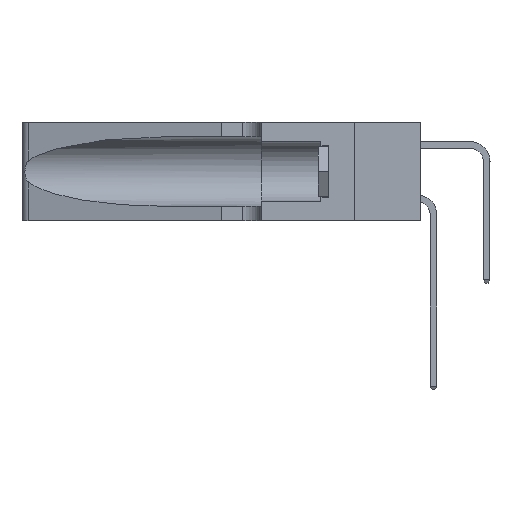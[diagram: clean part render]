
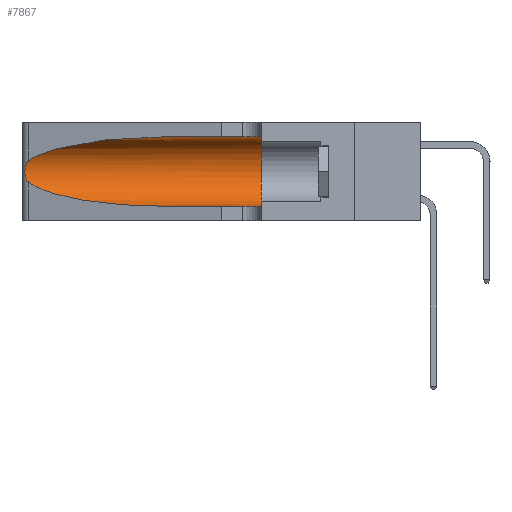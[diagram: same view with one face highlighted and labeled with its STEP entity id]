
A CAD part, left-side view. The second image highlights one B-rep face of the part: STEP entity #7867.
In plain terms, the highlighted cylindrical face has radius 3.308 mm (diameter 6.617 mm), a partial arc.
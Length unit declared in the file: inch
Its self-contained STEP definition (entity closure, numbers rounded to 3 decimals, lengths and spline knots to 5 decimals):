
#115 = CARTESIAN_POINT ( 'NONE',  ( 0.1305, 0.72297, 0.31525 ) ) ;
#390 = B_SPLINE_CURVE_WITH_KNOTS ( 'NONE', 3,
 ( #10693, #12631, #2793, #16438, #4817, #18344, #6835, #20268, #8833, #22129, #10775, #24006, #12704, #839 ),
 .UNSPECIFIED., .F., .F.,
 ( 4, 2, 2, 2, 2, 2, 4 ),
 ( 0., 0.00027, 0.00053, 0.00107, 0.0016, 0.00187, 0.00214 ),
 .UNSPECIFIED. ) ;
#839 = CARTESIAN_POINT ( 'NONE',  ( 0.25487, 1.22718, 0.14631 ) ) ;
#1038 = EDGE_CURVE ( 'NONE', #15591, #4184, #21441, .T. ) ;
#1065 =( BOUNDED_CURVE ( )  B_SPLINE_CURVE ( 3, ( #23646, #10409, #14245, #2492 ),
 .UNSPECIFIED., .F., .T. ) 
 B_SPLINE_CURVE_WITH_KNOTS ( ( 4, 4 ),
 ( 1.5708, 2.84003 ),
 .UNSPECIFIED. ) 
 CURVE ( )  GEOMETRIC_REPRESENTATION_ITEM ( )  RATIONAL_B_SPLINE_CURVE ( ( 1., 0.87, 0.87, 1. ) ) 
 REPRESENTATION_ITEM ( '' )  );
#2492 = CARTESIAN_POINT ( 'NONE',  ( 0.25487, 1.22718, 0.22369 ) ) ;
#2641 = CARTESIAN_POINT ( 'NONE',  ( 0.25487, 1.22718, 0.14631 ) ) ;
#2793 = CARTESIAN_POINT ( 'NONE',  ( 0.25639, 1.23184, 0.21858 ) ) ;
#2945 = DIRECTION ( 'NONE',  ( 0., 0., -1. ) ) ;
#3010 = EDGE_LOOP ( 'NONE', ( #16936, #16941, #18572, #11114, #23501, #21660 ) ) ;
#3634 =( BOUNDED_CURVE ( )  B_SPLINE_CURVE ( 3, ( #6744, #4717, #16345, #8723 ),
 .UNSPECIFIED., .F., .F. ) 
 B_SPLINE_CURVE_WITH_KNOTS ( ( 4, 4 ),
 ( 3.44316, 4.71239 ),
 .UNSPECIFIED. ) 
 CURVE ( )  GEOMETRIC_REPRESENTATION_ITEM ( )  RATIONAL_B_SPLINE_CURVE ( ( 1., 0.87, 0.87, 1. ) ) 
 REPRESENTATION_ITEM ( '' )  );
#4184 = VERTEX_POINT ( 'NONE', #13742 ) ;
#4603 = CARTESIAN_POINT ( 'NONE',  ( 0.1305, 1.61858, 0.31525 ) ) ;
#4717 = CARTESIAN_POINT ( 'NONE',  ( 0.2373, 1.15595, 0.08982 ) ) ;
#4817 = CARTESIAN_POINT ( 'NONE',  ( 0.25854, 1.2359, 0.20912 ) ) ;
#6711 = CARTESIAN_POINT ( 'NONE',  ( 0.25487, 1.22718, 0.22369 ) ) ;
#6723 = DIRECTION ( 'NONE',  ( 0., -1., 0. ) ) ;
#6744 = CARTESIAN_POINT ( 'NONE',  ( 0.25487, 1.22718, 0.14631 ) ) ;
#6835 = CARTESIAN_POINT ( 'NONE',  ( 0.26075, 1.23896, 0.19203 ) ) ;
#6985 = CARTESIAN_POINT ( 'NONE',  ( 0.1305, 1.61858, 0.185 ) ) ;
#7780 = EDGE_CURVE ( 'NONE', #24753, #19007, #3634, .T. ) ;
#7826 = CARTESIAN_POINT ( 'NONE',  ( 0.1305, 1.61858, 0.05475 ) ) ;
#7867 = ADVANCED_FACE ( 'NONE', ( #9242 ), #23777, .F. ) ;
#8723 = CARTESIAN_POINT ( 'NONE',  ( 0.1305, 0.72297, 0.05475 ) ) ;
#8833 = CARTESIAN_POINT ( 'NONE',  ( 0.26017, 1.23833, 0.17102 ) ) ;
#9125 = LINE ( 'NONE', #7826, #14219 ) ;
#9242 = FACE_OUTER_BOUND ( 'NONE', #3010, .T. ) ;
#10113 = EDGE_CURVE ( 'NONE', #19007, #4184, #9125, .T. ) ;
#10244 = VERTEX_POINT ( 'NONE', #115 ) ;
#10409 = CARTESIAN_POINT ( 'NONE',  ( 0.18966, 0.96281, 0.31525 ) ) ;
#10693 = CARTESIAN_POINT ( 'NONE',  ( 0.25487, 1.22718, 0.22369 ) ) ;
#10775 = CARTESIAN_POINT ( 'NONE',  ( 0.25789, 1.23486, 0.15765 ) ) ;
#11114 = ORIENTED_EDGE ( 'NONE', *, *, #10113, .T. ) ;
#11648 = CARTESIAN_POINT ( 'NONE',  ( 0.1305, 0.35, 0.31525 ) ) ;
#12631 = CARTESIAN_POINT ( 'NONE',  ( 0.25555, 1.22994, 0.2215 ) ) ;
#12667 = VECTOR ( 'NONE', #6723, 39.37008 ) ;
#12704 = CARTESIAN_POINT ( 'NONE',  ( 0.25555, 1.22993, 0.14849 ) ) ;
#13742 = CARTESIAN_POINT ( 'NONE',  ( 0.1305, 0.35, 0.05475 ) ) ;
#14219 = VECTOR ( 'NONE', #23041, 39.37008 ) ;
#14245 = CARTESIAN_POINT ( 'NONE',  ( 0.2373, 1.15595, 0.28018 ) ) ;
#15170 = EDGE_CURVE ( 'NONE', #10244, #17202, #1065, .T. ) ;
#15591 = VERTEX_POINT ( 'NONE', #11648 ) ;
#16345 = CARTESIAN_POINT ( 'NONE',  ( 0.18966, 0.96281, 0.05475 ) ) ;
#16438 = CARTESIAN_POINT ( 'NONE',  ( 0.25787, 1.23484, 0.2124 ) ) ;
#16543 = DIRECTION ( 'NONE',  ( 0., 0., 1. ) ) ;
#16936 = ORIENTED_EDGE ( 'NONE', *, *, #15170, .T. ) ;
#16941 = ORIENTED_EDGE ( 'NONE', *, *, #23113, .T. ) ;
#17202 = VERTEX_POINT ( 'NONE', #6711 ) ;
#17725 = LINE ( 'NONE', #4603, #12667 ) ;
#18344 = CARTESIAN_POINT ( 'NONE',  ( 0.26018, 1.23835, 0.19895 ) ) ;
#18572 = ORIENTED_EDGE ( 'NONE', *, *, #7780, .T. ) ;
#19007 = VERTEX_POINT ( 'NONE', #23470 ) ;
#20268 = CARTESIAN_POINT ( 'NONE',  ( 0.26075, 1.23896, 0.178 ) ) ;
#20503 = EDGE_CURVE ( 'NONE', #10244, #15591, #17725, .T. ) ;
#21122 = CARTESIAN_POINT ( 'NONE',  ( 0.1305, 0.35, 0.185 ) ) ;
#21441 = CIRCLE ( 'NONE', #21827, 0.13025 ) ;
#21660 = ORIENTED_EDGE ( 'NONE', *, *, #20503, .F. ) ;
#21827 = AXIS2_PLACEMENT_3D ( 'NONE', #21122, #23125, #16543 ) ;
#22129 = CARTESIAN_POINT ( 'NONE',  ( 0.25856, 1.23593, 0.16098 ) ) ;
#23041 = DIRECTION ( 'NONE',  ( 0., -1., 0. ) ) ;
#23113 = EDGE_CURVE ( 'NONE', #17202, #24753, #390, .T. ) ;
#23125 = DIRECTION ( 'NONE',  ( 0., 1., 0. ) ) ;
#23470 = CARTESIAN_POINT ( 'NONE',  ( 0.1305, 0.72297, 0.05475 ) ) ;
#23501 = ORIENTED_EDGE ( 'NONE', *, *, #1038, .F. ) ;
#23646 = CARTESIAN_POINT ( 'NONE',  ( 0.1305, 0.72297, 0.31525 ) ) ;
#23777 = CYLINDRICAL_SURFACE ( 'NONE', #24846, 0.13025 ) ;
#24006 = CARTESIAN_POINT ( 'NONE',  ( 0.25639, 1.23186, 0.15144 ) ) ;
#24150 = DIRECTION ( 'NONE',  ( 0., -1., 0. ) ) ;
#24753 = VERTEX_POINT ( 'NONE', #2641 ) ;
#24846 = AXIS2_PLACEMENT_3D ( 'NONE', #6985, #24150, #2945 ) ;
